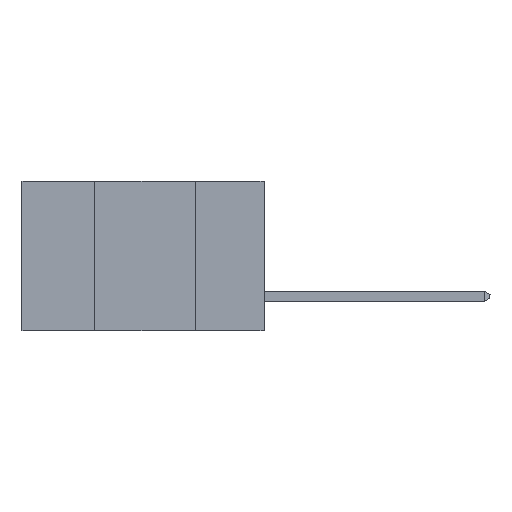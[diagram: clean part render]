
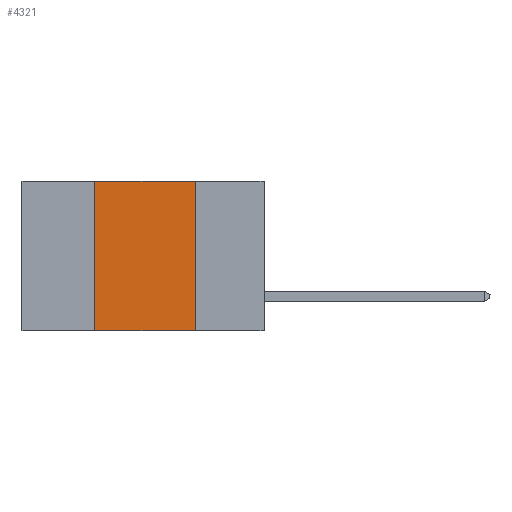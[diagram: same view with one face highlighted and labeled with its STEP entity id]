
A CAD part, left-side view. The second image highlights one B-rep face of the part: STEP entity #4321.
In plain terms, the highlighted planar face has unit normal (-1, 0, 0).
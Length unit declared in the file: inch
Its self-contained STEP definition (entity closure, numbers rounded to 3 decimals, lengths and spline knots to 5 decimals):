
#612 = DIRECTION ( 'NONE',  ( 1., 0., 0. ) ) ;
#659 = PLANE ( 'NONE',  #1083 ) ;
#663 = ORIENTED_EDGE ( 'NONE', *, *, #10654, .F. ) ;
#1083 = AXIS2_PLACEMENT_3D ( 'NONE', #13095, #612, #1735 ) ;
#1522 = ORIENTED_EDGE ( 'NONE', *, *, #1710, .F. ) ;
#1710 = EDGE_CURVE ( 'NONE', #2572, #11662, #10952, .T. ) ;
#1735 = DIRECTION ( 'NONE',  ( 0., 0., -1. ) ) ;
#2572 = VERTEX_POINT ( 'NONE', #5176 ) ;
#2848 = LINE ( 'NONE', #4149, #12832 ) ;
#2898 = VECTOR ( 'NONE', #3352, 39.37008 ) ;
#3352 = DIRECTION ( 'NONE',  ( 0., 0., 1. ) ) ;
#4149 = CARTESIAN_POINT ( 'NONE',  ( 0., 0.6, 0. ) ) ;
#4321 = ADVANCED_FACE ( 'NONE', ( #11742 ), #659, .F. ) ;
#5176 = CARTESIAN_POINT ( 'NONE',  ( 0., 0.17, 0. ) ) ;
#5976 = EDGE_CURVE ( 'NONE', #8549, #2572, #2848, .T. ) ;
#6010 = LINE ( 'NONE', #12574, #10932 ) ;
#6429 = CARTESIAN_POINT ( 'NONE',  ( 0., 0.42, -0.37 ) ) ;
#7446 = DIRECTION ( 'NONE',  ( 0., 0., -1. ) ) ;
#8144 = VECTOR ( 'NONE', #7446, 39.37008 ) ;
#8163 = ORIENTED_EDGE ( 'NONE', *, *, #9908, .T. ) ;
#8344 = DIRECTION ( 'NONE',  ( 0., -1., 0. ) ) ;
#8549 = VERTEX_POINT ( 'NONE', #10356 ) ;
#9681 = CARTESIAN_POINT ( 'NONE',  ( 0., 0.17, 0. ) ) ;
#9908 = EDGE_CURVE ( 'NONE', #12344, #11662, #6010, .T. ) ;
#10356 = CARTESIAN_POINT ( 'NONE',  ( 0., 0.42, 0. ) ) ;
#10565 = CARTESIAN_POINT ( 'NONE',  ( 0., 0.17, -0.37 ) ) ;
#10654 = EDGE_CURVE ( 'NONE', #12344, #8549, #11575, .T. ) ;
#10725 = CARTESIAN_POINT ( 'NONE',  ( 0., 0.42, 0. ) ) ;
#10932 = VECTOR ( 'NONE', #12440, 39.37008 ) ;
#10952 = LINE ( 'NONE', #9681, #8144 ) ;
#11575 = LINE ( 'NONE', #10725, #2898 ) ;
#11662 = VERTEX_POINT ( 'NONE', #10565 ) ;
#11742 = FACE_OUTER_BOUND ( 'NONE', #13050, .T. ) ;
#12176 = ORIENTED_EDGE ( 'NONE', *, *, #5976, .F. ) ;
#12344 = VERTEX_POINT ( 'NONE', #6429 ) ;
#12440 = DIRECTION ( 'NONE',  ( 0., -1., 0. ) ) ;
#12574 = CARTESIAN_POINT ( 'NONE',  ( 0., 0.6, -0.37 ) ) ;
#12832 = VECTOR ( 'NONE', #8344, 39.37008 ) ;
#13050 = EDGE_LOOP ( 'NONE', ( #1522, #12176, #663, #8163 ) ) ;
#13095 = CARTESIAN_POINT ( 'NONE',  ( 0., 0.6, 0. ) ) ;
